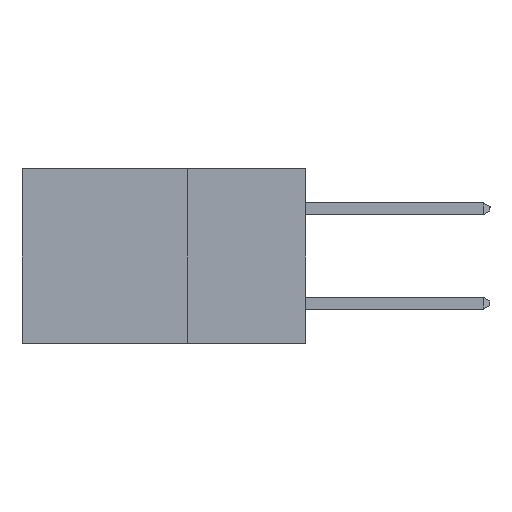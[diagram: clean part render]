
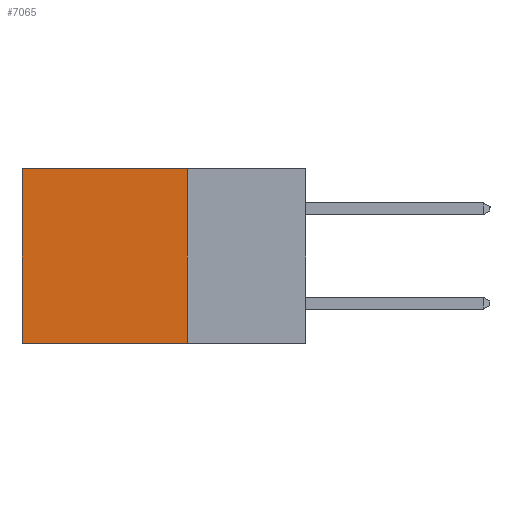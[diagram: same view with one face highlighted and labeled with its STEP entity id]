
A CAD part, left-side view. The second image highlights one B-rep face of the part: STEP entity #7065.
In plain terms, the highlighted planar face has unit normal (-1, 0, 0).
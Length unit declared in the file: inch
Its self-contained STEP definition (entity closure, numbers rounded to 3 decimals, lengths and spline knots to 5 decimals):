
#1153 = EDGE_CURVE ( 'NONE', #17051, #25431, #15553, .T. ) ;
#1600 = CARTESIAN_POINT ( 'NONE',  ( 0.2615, 0.25, -0.37 ) ) ;
#4657 = DIRECTION ( 'NONE',  ( 0., 1., 0. ) ) ;
#4774 = ORIENTED_EDGE ( 'NONE', *, *, #1153, .F. ) ;
#5544 = CARTESIAN_POINT ( 'NONE',  ( 0.2615, 0.25, 0. ) ) ;
#6341 = CARTESIAN_POINT ( 'NONE',  ( 0.2615, 0.6, -0.37 ) ) ;
#6660 = LINE ( 'NONE', #15056, #12862 ) ;
#6696 = EDGE_CURVE ( 'NONE', #9044, #18363, #25883, .T. ) ;
#7065 = ADVANCED_FACE ( 'NONE', ( #10308 ), #7964, .F. ) ;
#7964 = PLANE ( 'NONE',  #22003 ) ;
#9044 = VERTEX_POINT ( 'NONE', #5544 ) ;
#10129 = CARTESIAN_POINT ( 'NONE',  ( 0.2615, 0.6, 0. ) ) ;
#10308 = FACE_OUTER_BOUND ( 'NONE', #19555, .T. ) ;
#10429 = DIRECTION ( 'NONE',  ( 1., 0., 0. ) ) ;
#11068 = DIRECTION ( 'NONE',  ( 0., 0., -1. ) ) ;
#12630 = DIRECTION ( 'NONE',  ( 0., 0., -1. ) ) ;
#12862 = VECTOR ( 'NONE', #11068, 39.37008 ) ;
#13047 = ORIENTED_EDGE ( 'NONE', *, *, #18673, .F. ) ;
#13062 = VECTOR ( 'NONE', #26573, 39.37008 ) ;
#13751 = CARTESIAN_POINT ( 'NONE',  ( 0.2615, 0.25, -0.37 ) ) ;
#14744 = DIRECTION ( 'NONE',  ( 0., 0., -1. ) ) ;
#15056 = CARTESIAN_POINT ( 'NONE',  ( 0.2615, 0.25, -0.37 ) ) ;
#15553 = LINE ( 'NONE', #13751, #13062 ) ;
#16303 = EDGE_CURVE ( 'NONE', #18363, #25431, #22863, .T. ) ;
#17051 = VERTEX_POINT ( 'NONE', #17725 ) ;
#17725 = CARTESIAN_POINT ( 'NONE',  ( 0.2615, 0.25, -0.37 ) ) ;
#18363 = VERTEX_POINT ( 'NONE', #10129 ) ;
#18507 = VECTOR ( 'NONE', #14744, 39.37008 ) ;
#18673 = EDGE_CURVE ( 'NONE', #9044, #17051, #6660, .T. ) ;
#19555 = EDGE_LOOP ( 'NONE', ( #25704, #4774, #13047, #24681 ) ) ;
#22003 = AXIS2_PLACEMENT_3D ( 'NONE', #1600, #10429, #12630 ) ;
#22355 = CARTESIAN_POINT ( 'NONE',  ( 0.2615, 0.6, -0.37 ) ) ;
#22863 = LINE ( 'NONE', #6341, #18507 ) ;
#24204 = VECTOR ( 'NONE', #4657, 39.37008 ) ;
#24681 = ORIENTED_EDGE ( 'NONE', *, *, #6696, .T. ) ;
#25431 = VERTEX_POINT ( 'NONE', #22355 ) ;
#25481 = CARTESIAN_POINT ( 'NONE',  ( 0.2615, 0.25, 0. ) ) ;
#25704 = ORIENTED_EDGE ( 'NONE', *, *, #16303, .T. ) ;
#25883 = LINE ( 'NONE', #25481, #24204 ) ;
#26573 = DIRECTION ( 'NONE',  ( 0., 1., 0. ) ) ;
